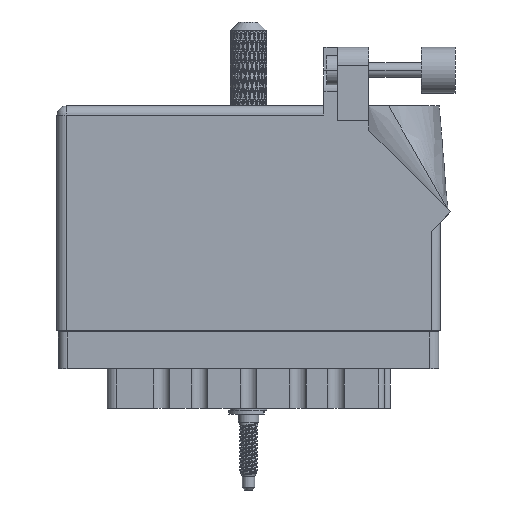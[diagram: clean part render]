
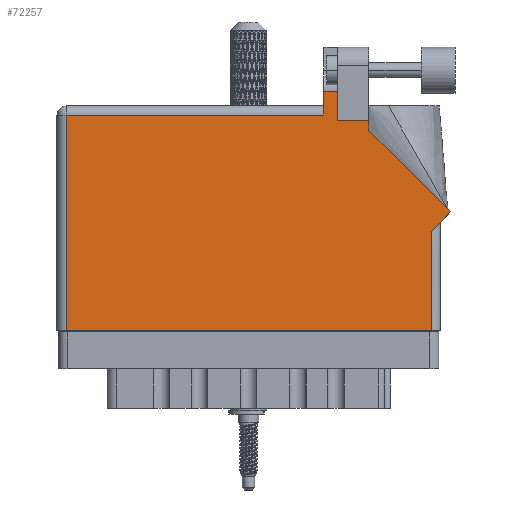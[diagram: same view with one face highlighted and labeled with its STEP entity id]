
A CAD part, front view. The second image highlights one B-rep face of the part: STEP entity #72257.
In plain terms, the highlighted face is planar.
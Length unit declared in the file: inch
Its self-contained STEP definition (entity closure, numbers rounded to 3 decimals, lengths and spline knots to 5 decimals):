
#6290 = DIRECTION ( 'NONE',  ( -1., 0., 0. ) ) ;
#12596 = ORIENTED_EDGE ( 'NONE', *, *, #80543, .T. ) ;
#12696 = VECTOR ( 'NONE', #106348, 39.37008 ) ;
#13078 = EDGE_CURVE ( 'NONE', #67999, #16567, #74496, .T. ) ;
#14051 = VECTOR ( 'NONE', #107756, 39.37008 ) ;
#15343 = DIRECTION ( 'NONE',  ( 0.707, 0.707, 0. ) ) ;
#15498 = CARTESIAN_POINT ( 'NONE',  ( 1.819, 1.468, 0. ) ) ;
#16567 = VERTEX_POINT ( 'NONE', #93308 ) ;
#17278 = EDGE_CURVE ( 'NONE', #50939, #71375, #29782, .T. ) ;
#18017 = DIRECTION ( 'NONE',  ( 0., -1., 0. ) ) ;
#18209 = CARTESIAN_POINT ( 'NONE',  ( 2.126, 1.43, 0. ) ) ;
#18618 = VERTEX_POINT ( 'NONE', #79320 ) ;
#19664 = LINE ( 'NONE', #97809, #109214 ) ;
#21566 = VECTOR ( 'NONE', #18017, 39.37008 ) ;
#23086 = EDGE_CURVE ( 'NONE', #31282, #67999, #114165, .T. ) ;
#23988 = VECTOR ( 'NONE', #31788, 39.37008 ) ;
#24291 = VECTOR ( 'NONE', #107819, 39.37008 ) ;
#29782 = LINE ( 'NONE', #114425, #23988 ) ;
#31271 = AXIS2_PLACEMENT_3D ( 'NONE', #48537, #77113, #112984 ) ;
#31282 = VERTEX_POINT ( 'NONE', #82384 ) ;
#31788 = DIRECTION ( 'NONE',  ( -1., 0., 0. ) ) ;
#32297 = DIRECTION ( 'NONE',  ( 1., 0., 0. ) ) ;
#38223 = DIRECTION ( 'NONE',  ( 0., 1., 0. ) ) ;
#41792 = CARTESIAN_POINT ( 'NONE',  ( 2.55, 0.675, 0. ) ) ;
#43349 = LINE ( 'NONE', #46410, #21566 ) ;
#43610 = CARTESIAN_POINT ( 'NONE',  ( 2.24377, 1.6315, 0. ) ) ;
#44413 = EDGE_LOOP ( 'NONE', ( #109871, #118377, #109181, #57389, #98782, #50920, #70882, #81188, #12596, #45398, #60646 ) ) ;
#45398 = ORIENTED_EDGE ( 'NONE', *, *, #69936, .T. ) ;
#45985 = CARTESIAN_POINT ( 'NONE',  ( 1.913, 1.43, 0. ) ) ;
#46410 = CARTESIAN_POINT ( 'NONE',  ( 1.819, 1.53, 0. ) ) ;
#47092 = VECTOR ( 'NONE', #32297, 39.37008 ) ;
#48537 = CARTESIAN_POINT ( 'NONE',  ( 0., 1.53, 0. ) ) ;
#48900 = LINE ( 'NONE', #61871, #24291 ) ;
#50920 = ORIENTED_EDGE ( 'NONE', *, *, #13078, .T. ) ;
#50939 = VERTEX_POINT ( 'NONE', #18209 ) ;
#53126 = VERTEX_POINT ( 'NONE', #41792 ) ;
#55087 = VECTOR ( 'NONE', #56995, 39.37008 ) ;
#56995 = DIRECTION ( 'NONE',  ( 0., -1., 0. ) ) ;
#57389 = ORIENTED_EDGE ( 'NONE', *, *, #111391, .T. ) ;
#60646 = ORIENTED_EDGE ( 'NONE', *, *, #17278, .T. ) ;
#61518 = CARTESIAN_POINT ( 'NONE',  ( 1.913, 1.6315, 0. ) ) ;
#61871 = CARTESIAN_POINT ( 'NONE',  ( 2.55, 0.737, 0. ) ) ;
#64207 = VECTOR ( 'NONE', #80723, 39.37008 ) ;
#64687 = LINE ( 'NONE', #70972, #77671 ) ;
#66431 = EDGE_CURVE ( 'NONE', #72200, #91140, #43349, .T. ) ;
#67999 = VERTEX_POINT ( 'NONE', #93780 ) ;
#69936 = EDGE_CURVE ( 'NONE', #101194, #50939, #97906, .T. ) ;
#70882 = ORIENTED_EDGE ( 'NONE', *, *, #98098, .T. ) ;
#70972 = CARTESIAN_POINT ( 'NONE',  ( 0., 1.468, 0. ) ) ;
#71375 = VERTEX_POINT ( 'NONE', #45985 ) ;
#72200 = VERTEX_POINT ( 'NONE', #100537 ) ;
#72257 = ADVANCED_FACE ( 'NONE', ( #78811 ), #76317, .F. ) ;
#74496 = LINE ( 'NONE', #87167, #47092 ) ;
#76317 = PLANE ( 'NONE',  #31271 ) ;
#76791 = EDGE_CURVE ( 'NONE', #71375, #85915, #118542, .T. ) ;
#77113 = DIRECTION ( 'NONE',  ( 0., 0., -1. ) ) ;
#77671 = VECTOR ( 'NONE', #6290, 39.37008 ) ;
#78581 = CARTESIAN_POINT ( 'NONE',  ( 2.68271, 0.80771, 0. ) ) ;
#78811 = FACE_OUTER_BOUND ( 'NONE', #44413, .T. ) ;
#79320 = CARTESIAN_POINT ( 'NONE',  ( 2.68271, 0.80771, 0. ) ) ;
#80543 = EDGE_CURVE ( 'NONE', #18618, #101194, #110946, .T. ) ;
#80723 = DIRECTION ( 'NONE',  ( -1., 0., 0. ) ) ;
#81188 = ORIENTED_EDGE ( 'NONE', *, *, #118964, .T. ) ;
#82384 = CARTESIAN_POINT ( 'NONE',  ( 0.062, 1.468, 0. ) ) ;
#85915 = VERTEX_POINT ( 'NONE', #61518 ) ;
#85918 = LINE ( 'NONE', #43610, #64207 ) ;
#87167 = CARTESIAN_POINT ( 'NONE',  ( 0., 0., 0. ) ) ;
#88461 = CARTESIAN_POINT ( 'NONE',  ( 2.126, 1.36442, 0. ) ) ;
#88567 = EDGE_CURVE ( 'NONE', #85915, #72200, #85918, .T. ) ;
#91140 = VERTEX_POINT ( 'NONE', #15498 ) ;
#93308 = CARTESIAN_POINT ( 'NONE',  ( 2.55, 0., 0. ) ) ;
#93444 = CARTESIAN_POINT ( 'NONE',  ( 1.913, 1.43, 0. ) ) ;
#93780 = CARTESIAN_POINT ( 'NONE',  ( 0.062, 0., 0. ) ) ;
#94540 = CARTESIAN_POINT ( 'NONE',  ( 0.062, 0., 0. ) ) ;
#97809 = CARTESIAN_POINT ( 'NONE',  ( 2.612, 0.737, 0. ) ) ;
#97906 = LINE ( 'NONE', #88461, #14051 ) ;
#98098 = EDGE_CURVE ( 'NONE', #16567, #53126, #48900, .T. ) ;
#98782 = ORIENTED_EDGE ( 'NONE', *, *, #23086, .T. ) ;
#100537 = CARTESIAN_POINT ( 'NONE',  ( 1.819, 1.6315, 0. ) ) ;
#101194 = VERTEX_POINT ( 'NONE', #103591 ) ;
#103591 = CARTESIAN_POINT ( 'NONE',  ( 2.126, 1.36442, 0. ) ) ;
#106348 = DIRECTION ( 'NONE',  ( -0.707, 0.707, 0. ) ) ;
#107756 = DIRECTION ( 'NONE',  ( 0., 1., 0. ) ) ;
#107819 = DIRECTION ( 'NONE',  ( 0., 1., 0. ) ) ;
#109181 = ORIENTED_EDGE ( 'NONE', *, *, #66431, .T. ) ;
#109214 = VECTOR ( 'NONE', #15343, 39.37008 ) ;
#109871 = ORIENTED_EDGE ( 'NONE', *, *, #76791, .T. ) ;
#110946 = LINE ( 'NONE', #78581, #12696 ) ;
#111391 = EDGE_CURVE ( 'NONE', #91140, #31282, #64687, .T. ) ;
#112984 = DIRECTION ( 'NONE',  ( -1., 0., 0. ) ) ;
#114165 = LINE ( 'NONE', #94540, #55087 ) ;
#114425 = CARTESIAN_POINT ( 'NONE',  ( 2.126, 1.43, 0. ) ) ;
#115694 = VECTOR ( 'NONE', #38223, 39.37008 ) ;
#118377 = ORIENTED_EDGE ( 'NONE', *, *, #88567, .T. ) ;
#118542 = LINE ( 'NONE', #93444, #115694 ) ;
#118964 = EDGE_CURVE ( 'NONE', #53126, #18618, #19664, .T. ) ;
